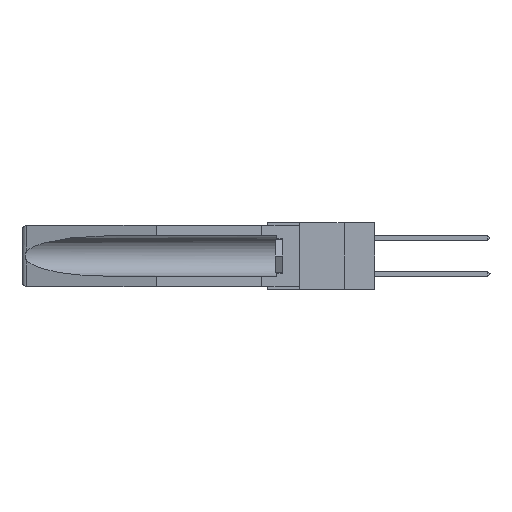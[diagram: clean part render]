
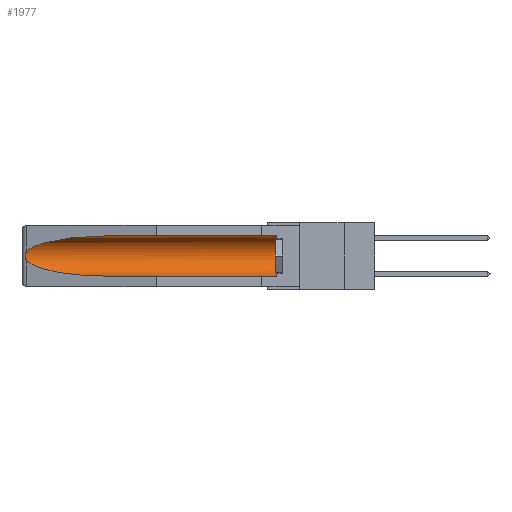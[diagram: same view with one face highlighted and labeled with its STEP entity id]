
A CAD part, left-side view. The second image highlights one B-rep face of the part: STEP entity #1977.
In plain terms, the highlighted cylindrical face has radius 2.857 mm (diameter 5.715 mm), a partial arc.
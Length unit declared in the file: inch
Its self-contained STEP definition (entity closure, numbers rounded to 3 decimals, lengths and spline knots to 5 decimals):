
#596 = DIRECTION ( 'NONE',  ( 0., 0., 1. ) ) ;
#869 = DIRECTION ( 'NONE',  ( 0., 1., 0. ) ) ;
#989 = FACE_OUTER_BOUND ( 'NONE', #21018, .T. ) ;
#1977 = ADVANCED_FACE ( 'NONE', ( #989 ), #23512, .F. ) ;
#2999 = ORIENTED_EDGE ( 'NONE', *, *, #7247, .T. ) ;
#3497 = CARTESIAN_POINT ( 'NONE',  ( 0.2673, 1.53269, -0.17917 ) ) ;
#3610 = CARTESIAN_POINT ( 'NONE',  ( 0.2673, 1.5327, -0.16383 ) ) ;
#4133 = CARTESIAN_POINT ( 'NONE',  ( 0.155, 0.126, -0.059 ) ) ;
#4572 = ORIENTED_EDGE ( 'NONE', *, *, #19015, .T. ) ;
#4663 = CARTESIAN_POINT ( 'NONE',  ( 0.26537, 1.52718, -0.14972 ) ) ;
#4961 =( BOUNDED_CURVE ( )  B_SPLINE_CURVE ( 3, ( #20341, #9565, #28248, #7060 ),
 .UNSPECIFIED., .F., .F. ) 
 B_SPLINE_CURVE_WITH_KNOTS ( ( 4, 4 ),
 ( 0.1948, 1.5708 ),
 .UNSPECIFIED. ) 
 CURVE ( )  GEOMETRIC_REPRESENTATION_ITEM ( )  RATIONAL_B_SPLINE_CURVE ( ( 1., 0.848, 0.848, 1. ) ) 
 REPRESENTATION_ITEM ( '' )  );
#5410 = CARTESIAN_POINT ( 'NONE',  ( 0.21114, 1.30732, -0.059 ) ) ;
#5963 = DIRECTION ( 'NONE',  ( 0., -1., 0. ) ) ;
#6040 = CARTESIAN_POINT ( 'NONE',  ( 0.155, -0.30754, -0.1715 ) ) ;
#6075 = CARTESIAN_POINT ( 'NONE',  ( 0.155, 0.126, -0.1715 ) ) ;
#7060 = CARTESIAN_POINT ( 'NONE',  ( 0.155, 1.07973, -0.284 ) ) ;
#7247 = EDGE_CURVE ( 'NONE', #29183, #30001, #15219, .T. ) ;
#7814 = CARTESIAN_POINT ( 'NONE',  ( 0.25451, 1.48313, -0.09465 ) ) ;
#7944 = CIRCLE ( 'NONE', #30334, 0.1125 ) ;
#8143 = CARTESIAN_POINT ( 'NONE',  ( 0.26537, 1.52718, -0.14972 ) ) ;
#8254 = VECTOR ( 'NONE', #31932, 39.37008 ) ;
#8585 = DIRECTION ( 'NONE',  ( 0., 0., 1. ) ) ;
#9340 = B_SPLINE_CURVE_WITH_KNOTS ( 'NONE', 3,
 ( #16407, #19039, #24316, #3610, #32203, #19145, #3497, #21794, #19258, #21908 ),
 .UNSPECIFIED., .F., .F.,
 ( 4, 2, 2, 2, 4 ),
 ( 0., 0.00029, 0.00058, 0.00087, 0.00117 ),
 .UNSPECIFIED. ) ;
#9565 = CARTESIAN_POINT ( 'NONE',  ( 0.25451, 1.48313, -0.24835 ) ) ;
#11005 = EDGE_CURVE ( 'NONE', #20698, #13058, #9340, .T. ) ;
#11455 = CARTESIAN_POINT ( 'NONE',  ( 0.155, -0.30754, -0.284 ) ) ;
#11626 = EDGE_CURVE ( 'NONE', #17624, #29183, #7944, .T. ) ;
#11990 = LINE ( 'NONE', #11455, #21051 ) ;
#13058 = VERTEX_POINT ( 'NONE', #18077 ) ;
#13614 = CARTESIAN_POINT ( 'NONE',  ( 0.155, -0.30754, -0.059 ) ) ;
#15219 = LINE ( 'NONE', #13614, #8254 ) ;
#16407 = CARTESIAN_POINT ( 'NONE',  ( 0.26537, 1.52718, -0.14972 ) ) ;
#17624 = VERTEX_POINT ( 'NONE', #22556 ) ;
#18077 = CARTESIAN_POINT ( 'NONE',  ( 0.26537, 1.52718, -0.19328 ) ) ;
#18451 = VERTEX_POINT ( 'NONE', #26385 ) ;
#18750 = ORIENTED_EDGE ( 'NONE', *, *, #20735, .T. ) ;
#19015 = EDGE_CURVE ( 'NONE', #30001, #20698, #33501, .T. ) ;
#19039 = CARTESIAN_POINT ( 'NONE',  ( 0.26597, 1.52961, -0.15275 ) ) ;
#19145 = CARTESIAN_POINT ( 'NONE',  ( 0.2675, 1.53308, -0.17534 ) ) ;
#19258 = CARTESIAN_POINT ( 'NONE',  ( 0.26597, 1.5296, -0.19026 ) ) ;
#20110 = ORIENTED_EDGE ( 'NONE', *, *, #30451, .F. ) ;
#20341 = CARTESIAN_POINT ( 'NONE',  ( 0.26537, 1.52718, -0.19328 ) ) ;
#20698 = VERTEX_POINT ( 'NONE', #4663 ) ;
#20735 = EDGE_CURVE ( 'NONE', #13058, #18451, #4961, .T. ) ;
#21002 = CARTESIAN_POINT ( 'NONE',  ( 0.155, 1.07973, -0.059 ) ) ;
#21018 = EDGE_LOOP ( 'NONE', ( #4572, #25224, #18750, #20110, #22793, #2999 ) ) ;
#21051 = VECTOR ( 'NONE', #869, 39.37008 ) ;
#21794 = CARTESIAN_POINT ( 'NONE',  ( 0.26655, 1.53094, -0.18657 ) ) ;
#21908 = CARTESIAN_POINT ( 'NONE',  ( 0.26537, 1.52718, -0.19328 ) ) ;
#22556 = CARTESIAN_POINT ( 'NONE',  ( 0.155, 0.126, -0.284 ) ) ;
#22793 = ORIENTED_EDGE ( 'NONE', *, *, #11626, .T. ) ;
#23512 = CYLINDRICAL_SURFACE ( 'NONE', #26229, 0.1125 ) ;
#24316 = CARTESIAN_POINT ( 'NONE',  ( 0.26654, 1.53092, -0.15636 ) ) ;
#25224 = ORIENTED_EDGE ( 'NONE', *, *, #11005, .T. ) ;
#26229 = AXIS2_PLACEMENT_3D ( 'NONE', #6040, #26872, #596 ) ;
#26385 = CARTESIAN_POINT ( 'NONE',  ( 0.155, 1.07973, -0.284 ) ) ;
#26872 = DIRECTION ( 'NONE',  ( 0., 1., 0. ) ) ;
#28248 = CARTESIAN_POINT ( 'NONE',  ( 0.21114, 1.30732, -0.284 ) ) ;
#29183 = VERTEX_POINT ( 'NONE', #4133 ) ;
#30001 = VERTEX_POINT ( 'NONE', #33779 ) ;
#30334 = AXIS2_PLACEMENT_3D ( 'NONE', #6075, #5963, #8585 ) ;
#30451 = EDGE_CURVE ( 'NONE', #17624, #18451, #11990, .T. ) ;
#31932 = DIRECTION ( 'NONE',  ( 0., 1., 0. ) ) ;
#32203 = CARTESIAN_POINT ( 'NONE',  ( 0.2675, 1.53308, -0.16763 ) ) ;
#33501 =( BOUNDED_CURVE ( )  B_SPLINE_CURVE ( 3, ( #21002, #5410, #7814, #8143 ),
 .UNSPECIFIED., .F., .F. ) 
 B_SPLINE_CURVE_WITH_KNOTS ( ( 4, 4 ),
 ( 4.71239, 6.08839 ),
 .UNSPECIFIED. ) 
 CURVE ( )  GEOMETRIC_REPRESENTATION_ITEM ( )  RATIONAL_B_SPLINE_CURVE ( ( 1., 0.848, 0.848, 1. ) ) 
 REPRESENTATION_ITEM ( '' )  );
#33779 = CARTESIAN_POINT ( 'NONE',  ( 0.155, 1.07973, -0.059 ) ) ;
